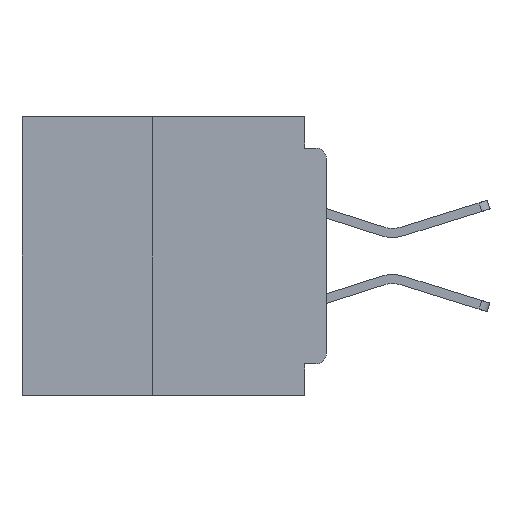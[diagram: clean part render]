
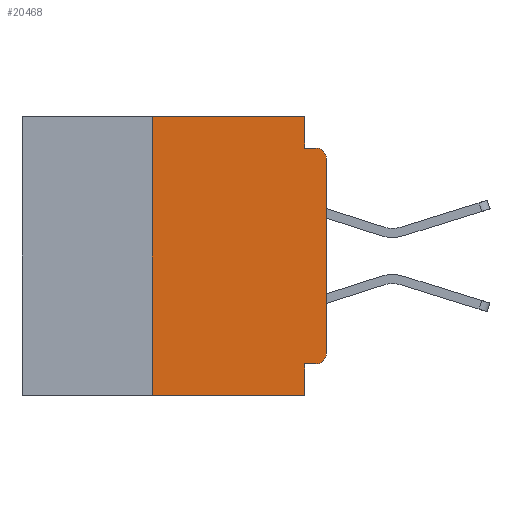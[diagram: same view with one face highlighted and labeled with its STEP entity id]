
A CAD part, left-side view. The second image highlights one B-rep face of the part: STEP entity #20468.
In plain terms, the highlighted planar face has unit normal (-1, 0, 0).
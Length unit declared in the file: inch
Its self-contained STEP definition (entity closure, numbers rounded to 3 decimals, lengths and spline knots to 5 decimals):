
#52 = EDGE_CURVE ( 'NONE', #41528, #42934, #21209, .T. ) ;
#55 = VERTEX_POINT ( 'NONE', #7163 ) ;
#1866 = EDGE_CURVE ( 'NONE', #41528, #55, #10325, .T. ) ;
#3049 = DIRECTION ( 'NONE',  ( 0., 0., 1. ) ) ;
#3261 = VERTEX_POINT ( 'NONE', #13722 ) ;
#3701 = ORIENTED_EDGE ( 'NONE', *, *, #25974, .T. ) ;
#4630 = DIRECTION ( 'NONE',  ( 0., -1., 0. ) ) ;
#4721 = CARTESIAN_POINT ( 'NONE',  ( 0., 0.437, 0. ) ) ;
#5330 = DIRECTION ( 'NONE',  ( 0., 1., 0. ) ) ;
#5786 = LINE ( 'NONE', #43687, #27279 ) ;
#6144 = AXIS2_PLACEMENT_3D ( 'NONE', #12475, #12298, #11994 ) ;
#6246 = CARTESIAN_POINT ( 'NONE',  ( 0., 0., -0.355 ) ) ;
#6315 = ORIENTED_EDGE ( 'NONE', *, *, #47051, .F. ) ;
#6979 = EDGE_CURVE ( 'NONE', #20265, #3261, #39269, .T. ) ;
#7163 = CARTESIAN_POINT ( 'NONE',  ( 0., 0., -0.34 ) ) ;
#7164 = DIRECTION ( 'NONE',  ( 0., 0., -1. ) ) ;
#7485 = DIRECTION ( 'NONE',  ( -1., 0., 0. ) ) ;
#7641 = CARTESIAN_POINT ( 'NONE',  ( 0., 0.25, -0.4 ) ) ;
#8133 = CARTESIAN_POINT ( 'NONE',  ( 0., 0.031, -0.4 ) ) ;
#8941 = VERTEX_POINT ( 'NONE', #7641 ) ;
#9542 = ORIENTED_EDGE ( 'NONE', *, *, #6979, .F. ) ;
#9629 = DIRECTION ( 'NONE',  ( 0., 0., 1. ) ) ;
#9960 = CARTESIAN_POINT ( 'NONE',  ( 0., 0.031, 0. ) ) ;
#10325 = CIRCLE ( 'NONE', #6144, 0.015 ) ;
#10545 = VERTEX_POINT ( 'NONE', #46459 ) ;
#11258 = CARTESIAN_POINT ( 'NONE',  ( 0., 0.437, 0. ) ) ;
#11926 = FACE_OUTER_BOUND ( 'NONE', #46351, .T. ) ;
#11994 = DIRECTION ( 'NONE',  ( 0., 0., -1. ) ) ;
#12298 = DIRECTION ( 'NONE',  ( -1., 0., 0. ) ) ;
#12475 = CARTESIAN_POINT ( 'NONE',  ( 0., 0.015, -0.34 ) ) ;
#13043 = CARTESIAN_POINT ( 'NONE',  ( 0., 0.437, -0.4 ) ) ;
#13722 = CARTESIAN_POINT ( 'NONE',  ( 0., 0.031, -0.045 ) ) ;
#13852 = ORIENTED_EDGE ( 'NONE', *, *, #35781, .F. ) ;
#15248 = AXIS2_PLACEMENT_3D ( 'NONE', #33259, #7485, #37573 ) ;
#15595 = EDGE_CURVE ( 'NONE', #8941, #10545, #44452, .T. ) ;
#16080 = VECTOR ( 'NONE', #21978, 39.37008 ) ;
#19070 = VECTOR ( 'NONE', #19102, 39.37008 ) ;
#19102 = DIRECTION ( 'NONE',  ( 0., 0., -1. ) ) ;
#19700 = CIRCLE ( 'NONE', #15248, 0.015 ) ;
#20265 = VERTEX_POINT ( 'NONE', #9960 ) ;
#20468 = ADVANCED_FACE ( 'NONE', ( #11926 ), #50027, .F. ) ;
#20536 = LINE ( 'NONE', #30906, #30620 ) ;
#20583 = VECTOR ( 'NONE', #4630, 39.37008 ) ;
#21209 = LINE ( 'NONE', #6246, #52829 ) ;
#21345 = EDGE_CURVE ( 'NONE', #8941, #51010, #32029, .T. ) ;
#21978 = DIRECTION ( 'NONE',  ( 0., -1., 0. ) ) ;
#24174 = EDGE_CURVE ( 'NONE', #3261, #41168, #5786, .T. ) ;
#25974 = EDGE_CURVE ( 'NONE', #50403, #41168, #19700, .T. ) ;
#26936 = AXIS2_PLACEMENT_3D ( 'NONE', #11258, #32934, #7164 ) ;
#27279 = VECTOR ( 'NONE', #39370, 39.37008 ) ;
#28036 = CARTESIAN_POINT ( 'NONE',  ( 0., 0., -0.06 ) ) ;
#28111 = EDGE_CURVE ( 'NONE', #55, #50403, #20536, .T. ) ;
#28871 = LINE ( 'NONE', #4721, #16080 ) ;
#28941 = ORIENTED_EDGE ( 'NONE', *, *, #21345, .T. ) ;
#30620 = VECTOR ( 'NONE', #9629, 39.37008 ) ;
#30906 = CARTESIAN_POINT ( 'NONE',  ( 0., 0., 0. ) ) ;
#32029 = LINE ( 'NONE', #13043, #20583 ) ;
#32075 = CARTESIAN_POINT ( 'NONE',  ( 0., 0.031, -0.355 ) ) ;
#32934 = DIRECTION ( 'NONE',  ( 1., 0., 0. ) ) ;
#33242 = ORIENTED_EDGE ( 'NONE', *, *, #24174, .F. ) ;
#33259 = CARTESIAN_POINT ( 'NONE',  ( 0., 0.015, -0.06 ) ) ;
#34311 = ORIENTED_EDGE ( 'NONE', *, *, #52, .F. ) ;
#35781 = EDGE_CURVE ( 'NONE', #42934, #51010, #51639, .T. ) ;
#36540 = ORIENTED_EDGE ( 'NONE', *, *, #28111, .T. ) ;
#36911 = CARTESIAN_POINT ( 'NONE',  ( 0., 0.015, -0.045 ) ) ;
#37573 = DIRECTION ( 'NONE',  ( 0., 0., -1. ) ) ;
#38210 = DIRECTION ( 'NONE',  ( 0., 0., -1. ) ) ;
#39269 = LINE ( 'NONE', #44869, #19070 ) ;
#39313 = CARTESIAN_POINT ( 'NONE',  ( 0., 0.031, -0.4 ) ) ;
#39370 = DIRECTION ( 'NONE',  ( 0., -1., 0. ) ) ;
#41168 = VERTEX_POINT ( 'NONE', #36911 ) ;
#41528 = VERTEX_POINT ( 'NONE', #47559 ) ;
#41568 = VECTOR ( 'NONE', #38210, 39.37008 ) ;
#42934 = VERTEX_POINT ( 'NONE', #32075 ) ;
#43096 = VECTOR ( 'NONE', #3049, 39.37008 ) ;
#43687 = CARTESIAN_POINT ( 'NONE',  ( 0., 0., -0.045 ) ) ;
#44452 = LINE ( 'NONE', #45909, #43096 ) ;
#44869 = CARTESIAN_POINT ( 'NONE',  ( 0., 0.031, 0. ) ) ;
#45909 = CARTESIAN_POINT ( 'NONE',  ( 0., 0.25, -0.4 ) ) ;
#46351 = EDGE_LOOP ( 'NONE', ( #36540, #3701, #33242, #9542, #6315, #49087, #28941, #13852, #34311, #54629 ) ) ;
#46459 = CARTESIAN_POINT ( 'NONE',  ( 0., 0.25, 0. ) ) ;
#47051 = EDGE_CURVE ( 'NONE', #10545, #20265, #28871, .T. ) ;
#47559 = CARTESIAN_POINT ( 'NONE',  ( 0., 0.015, -0.355 ) ) ;
#49087 = ORIENTED_EDGE ( 'NONE', *, *, #15595, .F. ) ;
#50027 = PLANE ( 'NONE',  #26936 ) ;
#50403 = VERTEX_POINT ( 'NONE', #28036 ) ;
#51010 = VERTEX_POINT ( 'NONE', #39313 ) ;
#51639 = LINE ( 'NONE', #8133, #41568 ) ;
#52829 = VECTOR ( 'NONE', #5330, 39.37008 ) ;
#54629 = ORIENTED_EDGE ( 'NONE', *, *, #1866, .T. ) ;
